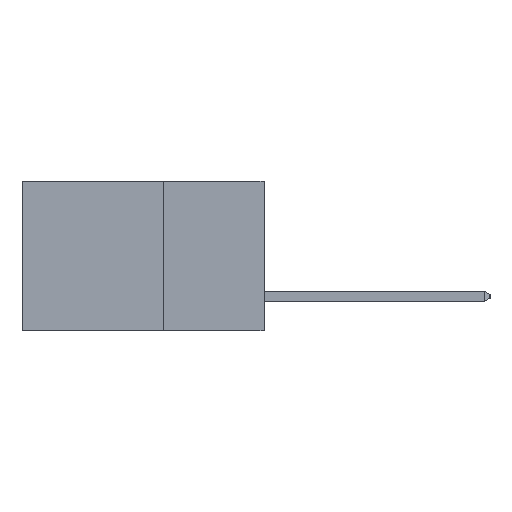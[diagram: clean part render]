
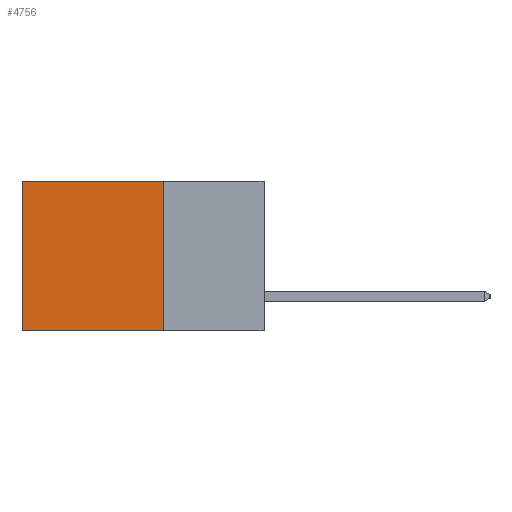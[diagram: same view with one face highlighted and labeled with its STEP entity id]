
A CAD part, left-side view. The second image highlights one B-rep face of the part: STEP entity #4756.
In plain terms, the highlighted planar face has unit normal (-1, 0, 0).
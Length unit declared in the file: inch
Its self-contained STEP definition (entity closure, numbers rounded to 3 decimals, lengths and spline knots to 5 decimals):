
#276 = ORIENTED_EDGE ( 'NONE', *, *, #13169, .T. ) ;
#709 = CARTESIAN_POINT ( 'NONE',  ( 0.2615, 0.25, -0.37 ) ) ;
#1835 = VECTOR ( 'NONE', #14009, 39.37008 ) ;
#2295 = VECTOR ( 'NONE', #9423, 39.37008 ) ;
#2445 = EDGE_CURVE ( 'NONE', #12693, #6636, #11153, .T. ) ;
#2580 = CARTESIAN_POINT ( 'NONE',  ( 0.2615, 0.6, -0.37 ) ) ;
#2630 = DIRECTION ( 'NONE',  ( 0., 1., 0. ) ) ;
#2687 = CARTESIAN_POINT ( 'NONE',  ( 0.2615, 0.25, 0. ) ) ;
#2985 = CARTESIAN_POINT ( 'NONE',  ( 0.2615, 0.25, 0. ) ) ;
#4194 = VERTEX_POINT ( 'NONE', #13306 ) ;
#4756 = ADVANCED_FACE ( 'NONE', ( #8175 ), #8248, .F. ) ;
#6366 = LINE ( 'NONE', #7882, #2295 ) ;
#6587 = VECTOR ( 'NONE', #2630, 39.37008 ) ;
#6636 = VERTEX_POINT ( 'NONE', #12394 ) ;
#7882 = CARTESIAN_POINT ( 'NONE',  ( 0.2615, 0.25, -0.37 ) ) ;
#8121 = DIRECTION ( 'NONE',  ( 0., 0., -1. ) ) ;
#8126 = DIRECTION ( 'NONE',  ( 1., 0., 0. ) ) ;
#8175 = FACE_OUTER_BOUND ( 'NONE', #15912, .T. ) ;
#8211 = ORIENTED_EDGE ( 'NONE', *, *, #13507, .F. ) ;
#8248 = PLANE ( 'NONE',  #18013 ) ;
#8324 = CARTESIAN_POINT ( 'NONE',  ( 0.2615, 0.25, -0.37 ) ) ;
#8366 = VERTEX_POINT ( 'NONE', #709 ) ;
#9423 = DIRECTION ( 'NONE',  ( 0., 0., -1. ) ) ;
#11153 = LINE ( 'NONE', #2687, #6587 ) ;
#11617 = ORIENTED_EDGE ( 'NONE', *, *, #2445, .T. ) ;
#12394 = CARTESIAN_POINT ( 'NONE',  ( 0.2615, 0.6, 0. ) ) ;
#12618 = VECTOR ( 'NONE', #14839, 39.37008 ) ;
#12693 = VERTEX_POINT ( 'NONE', #2985 ) ;
#13169 = EDGE_CURVE ( 'NONE', #6636, #4194, #17115, .T. ) ;
#13306 = CARTESIAN_POINT ( 'NONE',  ( 0.2615, 0.6, -0.37 ) ) ;
#13507 = EDGE_CURVE ( 'NONE', #12693, #8366, #6366, .T. ) ;
#14009 = DIRECTION ( 'NONE',  ( 0., 1., 0. ) ) ;
#14195 = EDGE_CURVE ( 'NONE', #8366, #4194, #18031, .T. ) ;
#14839 = DIRECTION ( 'NONE',  ( 0., 0., -1. ) ) ;
#15077 = ORIENTED_EDGE ( 'NONE', *, *, #14195, .F. ) ;
#15586 = CARTESIAN_POINT ( 'NONE',  ( 0.2615, 0.25, -0.37 ) ) ;
#15912 = EDGE_LOOP ( 'NONE', ( #276, #15077, #8211, #11617 ) ) ;
#17115 = LINE ( 'NONE', #2580, #12618 ) ;
#18013 = AXIS2_PLACEMENT_3D ( 'NONE', #8324, #8126, #8121 ) ;
#18031 = LINE ( 'NONE', #15586, #1835 ) ;
